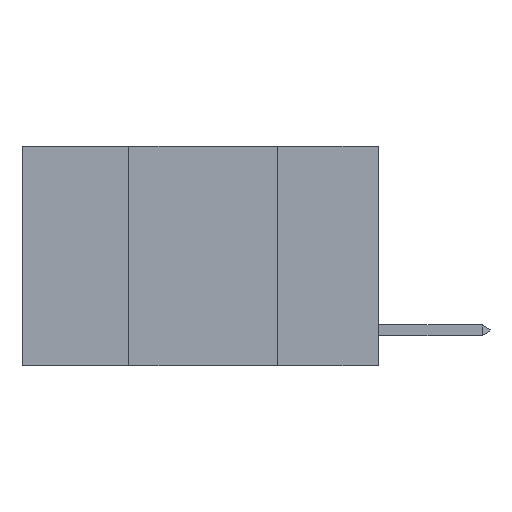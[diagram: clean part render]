
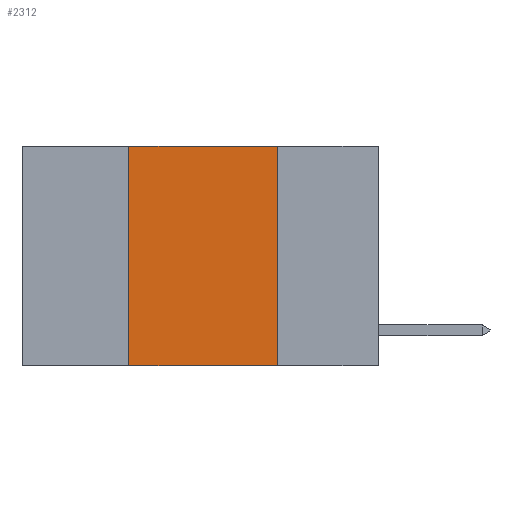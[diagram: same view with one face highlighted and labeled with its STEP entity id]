
A CAD part, left-side view. The second image highlights one B-rep face of the part: STEP entity #2312.
In plain terms, the highlighted planar face has unit normal (-1, 0, 0).
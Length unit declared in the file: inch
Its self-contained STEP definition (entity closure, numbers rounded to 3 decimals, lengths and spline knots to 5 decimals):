
#60 = EDGE_LOOP ( 'NONE', ( #2843, #18737, #18091, #7004 ) ) ;
#653 = CARTESIAN_POINT ( 'NONE',  ( 0., 0.6, 0. ) ) ;
#849 = DIRECTION ( 'NONE',  ( 0., 0., 1. ) ) ;
#2312 = ADVANCED_FACE ( 'NONE', ( #6067 ), #3827, .F. ) ;
#2843 = ORIENTED_EDGE ( 'NONE', *, *, #21444, .F. ) ;
#3273 = EDGE_CURVE ( 'NONE', #21565, #17568, #15459, .T. ) ;
#3398 = EDGE_CURVE ( 'NONE', #16128, #19457, #23239, .T. ) ;
#3827 = PLANE ( 'NONE',  #14003 ) ;
#4576 = DIRECTION ( 'NONE',  ( 0., 0., -1. ) ) ;
#5875 = CARTESIAN_POINT ( 'NONE',  ( 0., 0.6, 0. ) ) ;
#6067 = FACE_OUTER_BOUND ( 'NONE', #60, .T. ) ;
#6684 = VECTOR ( 'NONE', #25811, 39.37008 ) ;
#7004 = ORIENTED_EDGE ( 'NONE', *, *, #3398, .T. ) ;
#7952 = DIRECTION ( 'NONE',  ( 1., 0., 0. ) ) ;
#9267 = CARTESIAN_POINT ( 'NONE',  ( 0., 0.6, -0.37 ) ) ;
#10318 = VECTOR ( 'NONE', #849, 39.37008 ) ;
#10791 = CARTESIAN_POINT ( 'NONE',  ( 0., 0.17, 0. ) ) ;
#11554 = CARTESIAN_POINT ( 'NONE',  ( 0., 0.17, 0. ) ) ;
#13188 = CARTESIAN_POINT ( 'NONE',  ( 0., 0.42, 0. ) ) ;
#14003 = AXIS2_PLACEMENT_3D ( 'NONE', #5875, #7952, #22468 ) ;
#14500 = EDGE_CURVE ( 'NONE', #16128, #21565, #15200, .T. ) ;
#15200 = LINE ( 'NONE', #13188, #10318 ) ;
#15459 = LINE ( 'NONE', #653, #25856 ) ;
#16128 = VERTEX_POINT ( 'NONE', #17545 ) ;
#16788 = LINE ( 'NONE', #10791, #22291 ) ;
#17545 = CARTESIAN_POINT ( 'NONE',  ( 0., 0.42, -0.37 ) ) ;
#17568 = VERTEX_POINT ( 'NONE', #11554 ) ;
#18091 = ORIENTED_EDGE ( 'NONE', *, *, #14500, .F. ) ;
#18737 = ORIENTED_EDGE ( 'NONE', *, *, #3273, .F. ) ;
#19285 = DIRECTION ( 'NONE',  ( 0., -1., 0. ) ) ;
#19457 = VERTEX_POINT ( 'NONE', #21252 ) ;
#21252 = CARTESIAN_POINT ( 'NONE',  ( 0., 0.17, -0.37 ) ) ;
#21444 = EDGE_CURVE ( 'NONE', #17568, #19457, #16788, .T. ) ;
#21493 = CARTESIAN_POINT ( 'NONE',  ( 0., 0.42, 0. ) ) ;
#21565 = VERTEX_POINT ( 'NONE', #21493 ) ;
#22291 = VECTOR ( 'NONE', #4576, 39.37008 ) ;
#22468 = DIRECTION ( 'NONE',  ( 0., 0., -1. ) ) ;
#23239 = LINE ( 'NONE', #9267, #6684 ) ;
#25811 = DIRECTION ( 'NONE',  ( 0., -1., 0. ) ) ;
#25856 = VECTOR ( 'NONE', #19285, 39.37008 ) ;
